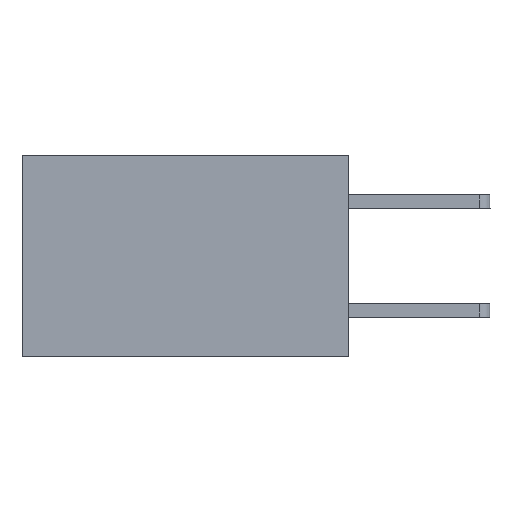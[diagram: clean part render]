
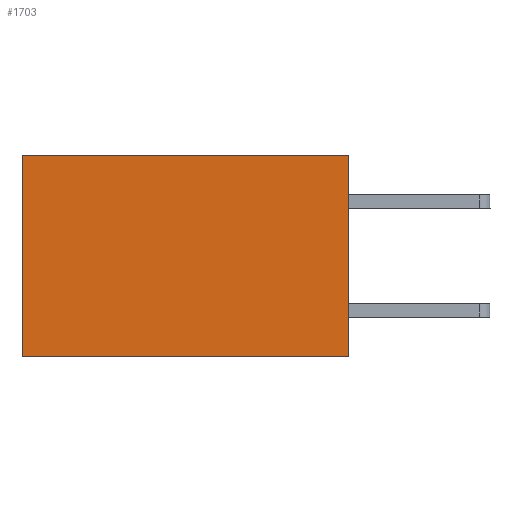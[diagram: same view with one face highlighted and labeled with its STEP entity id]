
A CAD part, left-side view. The second image highlights one B-rep face of the part: STEP entity #1703.
In plain terms, the highlighted planar face has unit normal (-1, 0, 0).
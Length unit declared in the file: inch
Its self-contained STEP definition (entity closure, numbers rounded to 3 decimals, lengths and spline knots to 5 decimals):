
#388 = CARTESIAN_POINT ( 'NONE',  ( 0.298, 0., -0.37 ) ) ;
#631 = DIRECTION ( 'NONE',  ( 0., 0., -1. ) ) ;
#731 = CARTESIAN_POINT ( 'NONE',  ( 0.298, 0., 0. ) ) ;
#974 = VERTEX_POINT ( 'NONE', #388 ) ;
#1360 = LINE ( 'NONE', #5398, #4581 ) ;
#1631 = PLANE ( 'NONE',  #3218 ) ;
#1703 = ADVANCED_FACE ( 'NONE', ( #3591 ), #1631, .F. ) ;
#1899 = VECTOR ( 'NONE', #7547, 39.37008 ) ;
#2443 = VERTEX_POINT ( 'NONE', #2656 ) ;
#2497 = CARTESIAN_POINT ( 'NONE',  ( 0.298, 0.6, -0.37 ) ) ;
#2656 = CARTESIAN_POINT ( 'NONE',  ( 0.298, 0.6, 0. ) ) ;
#3218 = AXIS2_PLACEMENT_3D ( 'NONE', #4395, #7140, #7860 ) ;
#3265 = ORIENTED_EDGE ( 'NONE', *, *, #4079, .T. ) ;
#3365 = DIRECTION ( 'NONE',  ( 0., 1., 0. ) ) ;
#3591 = FACE_OUTER_BOUND ( 'NONE', #7449, .T. ) ;
#3938 = VERTEX_POINT ( 'NONE', #7220 ) ;
#4079 = EDGE_CURVE ( 'NONE', #3938, #2443, #7010, .T. ) ;
#4395 = CARTESIAN_POINT ( 'NONE',  ( 0.298, 0., 0. ) ) ;
#4423 = VERTEX_POINT ( 'NONE', #2497 ) ;
#4581 = VECTOR ( 'NONE', #5362, 39.37008 ) ;
#4598 = EDGE_CURVE ( 'NONE', #2443, #4423, #5450, .T. ) ;
#4602 = VECTOR ( 'NONE', #3365, 39.37008 ) ;
#5362 = DIRECTION ( 'NONE',  ( 0., 1., 0. ) ) ;
#5398 = CARTESIAN_POINT ( 'NONE',  ( 0.298, 0., -0.37 ) ) ;
#5450 = LINE ( 'NONE', #8234, #1899 ) ;
#5898 = ORIENTED_EDGE ( 'NONE', *, *, #7293, .F. ) ;
#5911 = ORIENTED_EDGE ( 'NONE', *, *, #4598, .T. ) ;
#6033 = VECTOR ( 'NONE', #631, 39.37008 ) ;
#6312 = CARTESIAN_POINT ( 'NONE',  ( 0.298, 0., 0. ) ) ;
#6765 = LINE ( 'NONE', #731, #6033 ) ;
#7010 = LINE ( 'NONE', #6312, #4602 ) ;
#7140 = DIRECTION ( 'NONE',  ( 1., 0., 0. ) ) ;
#7220 = CARTESIAN_POINT ( 'NONE',  ( 0.298, 0., 0. ) ) ;
#7293 = EDGE_CURVE ( 'NONE', #974, #4423, #1360, .T. ) ;
#7449 = EDGE_LOOP ( 'NONE', ( #5911, #5898, #8596, #3265 ) ) ;
#7547 = DIRECTION ( 'NONE',  ( 0., 0., -1. ) ) ;
#7860 = DIRECTION ( 'NONE',  ( 0., 0., -1. ) ) ;
#8234 = CARTESIAN_POINT ( 'NONE',  ( 0.298, 0.6, 0. ) ) ;
#8565 = EDGE_CURVE ( 'NONE', #3938, #974, #6765, .T. ) ;
#8596 = ORIENTED_EDGE ( 'NONE', *, *, #8565, .F. ) ;
